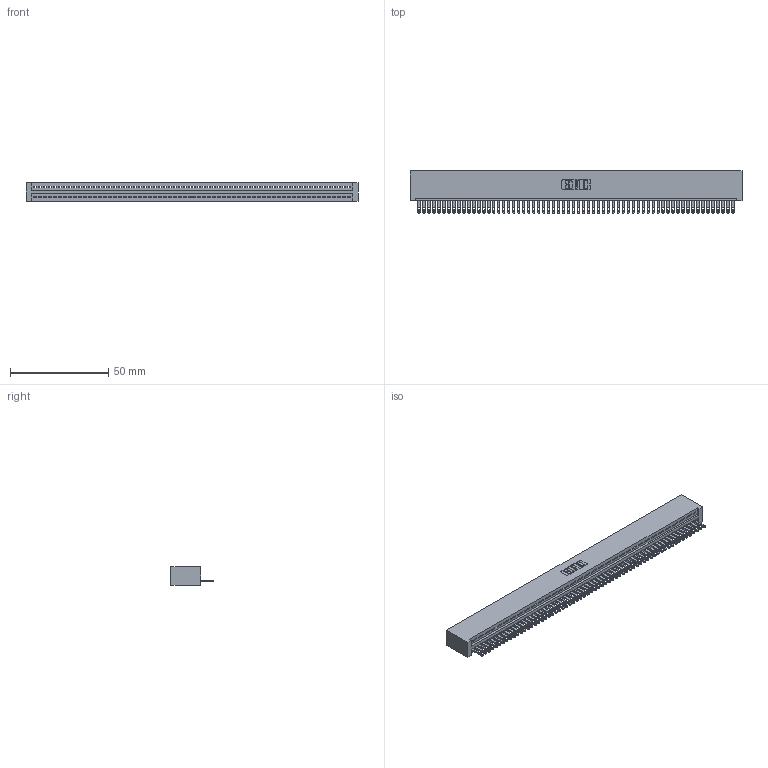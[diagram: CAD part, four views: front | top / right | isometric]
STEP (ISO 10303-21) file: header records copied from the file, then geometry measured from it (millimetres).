
FILE_DESCRIPTION (( 'STEP AP203' ), '1' );
FILE_NAME ('895-064-500-101.STEP', '2020-09-28T09:21:29', ( '' ), ( '' ), 'SwSTEP 2.0', 'SolidWorks 2020', '' );
FILE_SCHEMA (( 'CONFIG_CONTROL_DESIGN' ));
Length unit declared in the file: inch
Products named in the file (3): 345-292-001_345-293-100; 895-064-500-101; 845 Part_No Mounting Lugs
Assembly tree (65 placements, depth 2):
  895-064-500-101
    845 Part_No Mounting Lugs
    345-292-001_345-293-100  x64
Bounding box: 169.16 x 21.51 x 9.4 mm (x, y, z)
Volume: 16871.6 mm3; surface area: 23053.6 mm2
Topology: 65 solids, 65 shells, 3574 faces, 11069 edges, 7378 vertices
Faces by surface type: plane 2252, cylinder 1322
Entity records: 44859 total; most frequent: CARTESIAN_POINT 7776, ORIENTED_EDGE 7774, DIRECTION 6755, EDGE_CURVE 3887, VECTOR 3503, LINE 3503, VERTEX_POINT 2590, AXIS2_PLACEMENT_3D 1626
